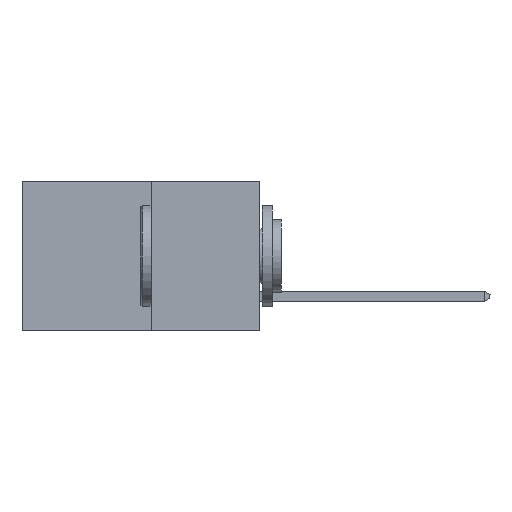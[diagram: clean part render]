
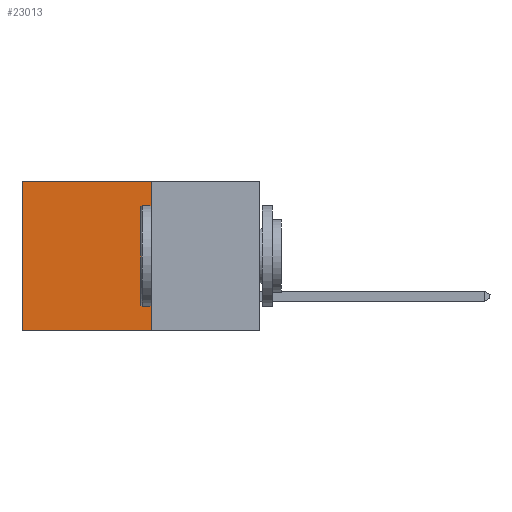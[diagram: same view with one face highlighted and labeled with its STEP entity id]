
A CAD part, left-side view. The second image highlights one B-rep face of the part: STEP entity #23013.
In plain terms, the highlighted planar face has unit normal (-1, 0, 0).
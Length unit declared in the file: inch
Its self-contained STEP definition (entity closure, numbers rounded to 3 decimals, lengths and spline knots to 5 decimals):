
#574 = DIRECTION ( 'NONE',  ( 0., 1., 0. ) ) ;
#1407 = DIRECTION ( 'NONE',  ( 0., 0., -1. ) ) ;
#2611 = VECTOR ( 'NONE', #574, 39.37008 ) ;
#2973 = VECTOR ( 'NONE', #21500, 39.37008 ) ;
#3055 = VERTEX_POINT ( 'NONE', #9978 ) ;
#5651 = CARTESIAN_POINT ( 'NONE',  ( 0.277, 0.27, -0.37 ) ) ;
#6231 = CARTESIAN_POINT ( 'NONE',  ( 0.277, 0.27, -0.37 ) ) ;
#6681 = VECTOR ( 'NONE', #1407, 39.37008 ) ;
#7293 = CARTESIAN_POINT ( 'NONE',  ( 0.277, 0.27, 0. ) ) ;
#7365 = EDGE_CURVE ( 'NONE', #22936, #18364, #9139, .T. ) ;
#7539 = DIRECTION ( 'NONE',  ( 0., 0., -1. ) ) ;
#7608 = LINE ( 'NONE', #6231, #2611 ) ;
#8065 = FACE_OUTER_BOUND ( 'NONE', #12095, .T. ) ;
#8653 = CARTESIAN_POINT ( 'NONE',  ( 0.277, 0.27, 0. ) ) ;
#8905 = VECTOR ( 'NONE', #21705, 39.37008 ) ;
#9139 = LINE ( 'NONE', #21612, #2973 ) ;
#9978 = CARTESIAN_POINT ( 'NONE',  ( 0.277, 0.59, 0. ) ) ;
#11440 = CARTESIAN_POINT ( 'NONE',  ( 0.277, 0.59, -0.37 ) ) ;
#12095 = EDGE_LOOP ( 'NONE', ( #18764, #17674, #24101, #21164 ) ) ;
#13316 = LINE ( 'NONE', #8653, #8905 ) ;
#15036 = VERTEX_POINT ( 'NONE', #11440 ) ;
#16849 = PLANE ( 'NONE',  #23947 ) ;
#17674 = ORIENTED_EDGE ( 'NONE', *, *, #19777, .F. ) ;
#18364 = VERTEX_POINT ( 'NONE', #19103 ) ;
#18721 = DIRECTION ( 'NONE',  ( 1., 0., 0. ) ) ;
#18764 = ORIENTED_EDGE ( 'NONE', *, *, #21534, .T. ) ;
#19103 = CARTESIAN_POINT ( 'NONE',  ( 0.277, 0.27, -0.37 ) ) ;
#19777 = EDGE_CURVE ( 'NONE', #18364, #15036, #7608, .T. ) ;
#21164 = ORIENTED_EDGE ( 'NONE', *, *, #23606, .T. ) ;
#21500 = DIRECTION ( 'NONE',  ( 0., 0., -1. ) ) ;
#21534 = EDGE_CURVE ( 'NONE', #3055, #15036, #21586, .T. ) ;
#21586 = LINE ( 'NONE', #23829, #6681 ) ;
#21612 = CARTESIAN_POINT ( 'NONE',  ( 0.277, 0.27, -0.37 ) ) ;
#21705 = DIRECTION ( 'NONE',  ( 0., 1., 0. ) ) ;
#22936 = VERTEX_POINT ( 'NONE', #7293 ) ;
#23013 = ADVANCED_FACE ( 'NONE', ( #8065 ), #16849, .F. ) ;
#23606 = EDGE_CURVE ( 'NONE', #22936, #3055, #13316, .T. ) ;
#23829 = CARTESIAN_POINT ( 'NONE',  ( 0.277, 0.59, -0.37 ) ) ;
#23947 = AXIS2_PLACEMENT_3D ( 'NONE', #5651, #18721, #7539 ) ;
#24101 = ORIENTED_EDGE ( 'NONE', *, *, #7365, .F. ) ;
